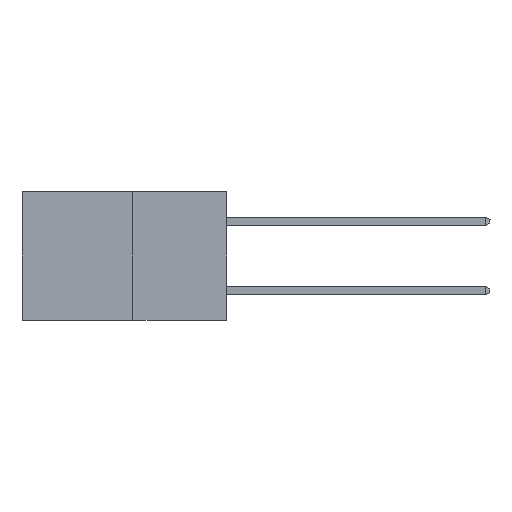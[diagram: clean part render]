
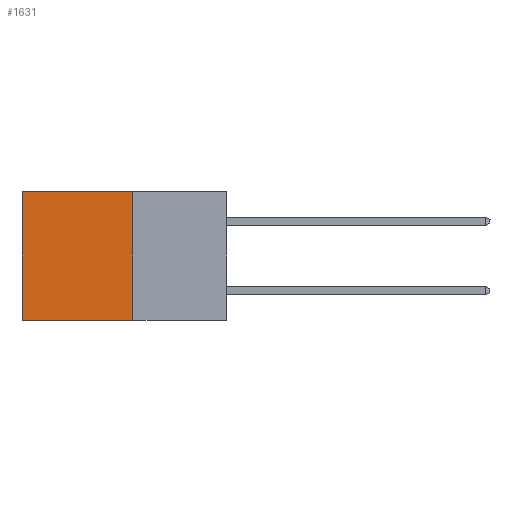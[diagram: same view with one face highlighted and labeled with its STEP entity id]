
A CAD part, left-side view. The second image highlights one B-rep face of the part: STEP entity #1631.
In plain terms, the highlighted planar face has unit normal (-1, 0, 0).
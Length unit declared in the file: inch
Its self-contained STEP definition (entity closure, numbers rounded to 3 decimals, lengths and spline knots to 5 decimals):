
#41 = ORIENTED_EDGE ( 'NONE', *, *, #3893, .F. ) ;
#108 = ORIENTED_EDGE ( 'NONE', *, *, #2217, .T. ) ;
#837 = CARTESIAN_POINT ( 'NONE',  ( 0.277, 0.59, -0.37 ) ) ;
#1186 = VERTEX_POINT ( 'NONE', #837 ) ;
#1601 = VECTOR ( 'NONE', #8735, 39.37008 ) ;
#1627 = ORIENTED_EDGE ( 'NONE', *, *, #11690, .T. ) ;
#1631 = ADVANCED_FACE ( 'NONE', ( #8624 ), #9342, .F. ) ;
#1676 = VECTOR ( 'NONE', #7526, 39.37008 ) ;
#1737 = AXIS2_PLACEMENT_3D ( 'NONE', #5653, #9213, #4136 ) ;
#2217 = EDGE_CURVE ( 'NONE', #6493, #3248, #7183, .T. ) ;
#2330 = CARTESIAN_POINT ( 'NONE',  ( 0.277, 0.59, 0. ) ) ;
#3174 = ORIENTED_EDGE ( 'NONE', *, *, #10283, .F. ) ;
#3248 = VERTEX_POINT ( 'NONE', #2330 ) ;
#3893 = EDGE_CURVE ( 'NONE', #6493, #13014, #9039, .T. ) ;
#4136 = DIRECTION ( 'NONE',  ( 0., 0., -1. ) ) ;
#4341 = LINE ( 'NONE', #9833, #7090 ) ;
#4366 = LINE ( 'NONE', #12512, #1601 ) ;
#5557 = CARTESIAN_POINT ( 'NONE',  ( 0.277, 0.27, -0.37 ) ) ;
#5637 = EDGE_LOOP ( 'NONE', ( #1627, #3174, #41, #108 ) ) ;
#5653 = CARTESIAN_POINT ( 'NONE',  ( 0.277, 0.27, -0.37 ) ) ;
#6493 = VERTEX_POINT ( 'NONE', #10559 ) ;
#7090 = VECTOR ( 'NONE', #9900, 39.37008 ) ;
#7183 = LINE ( 'NONE', #7540, #1676 ) ;
#7526 = DIRECTION ( 'NONE',  ( 0., 1., 0. ) ) ;
#7540 = CARTESIAN_POINT ( 'NONE',  ( 0.277, 0.27, 0. ) ) ;
#8395 = CARTESIAN_POINT ( 'NONE',  ( 0.277, 0.27, -0.37 ) ) ;
#8501 = DIRECTION ( 'NONE',  ( 0., 0., -1. ) ) ;
#8624 = FACE_OUTER_BOUND ( 'NONE', #5637, .T. ) ;
#8735 = DIRECTION ( 'NONE',  ( 0., 0., -1. ) ) ;
#9039 = LINE ( 'NONE', #8395, #11686 ) ;
#9213 = DIRECTION ( 'NONE',  ( 1., 0., 0. ) ) ;
#9342 = PLANE ( 'NONE',  #1737 ) ;
#9833 = CARTESIAN_POINT ( 'NONE',  ( 0.277, 0.27, -0.37 ) ) ;
#9900 = DIRECTION ( 'NONE',  ( 0., 1., 0. ) ) ;
#10283 = EDGE_CURVE ( 'NONE', #13014, #1186, #4341, .T. ) ;
#10559 = CARTESIAN_POINT ( 'NONE',  ( 0.277, 0.27, 0. ) ) ;
#11686 = VECTOR ( 'NONE', #8501, 39.37008 ) ;
#11690 = EDGE_CURVE ( 'NONE', #3248, #1186, #4366, .T. ) ;
#12512 = CARTESIAN_POINT ( 'NONE',  ( 0.277, 0.59, -0.37 ) ) ;
#13014 = VERTEX_POINT ( 'NONE', #5557 ) ;
